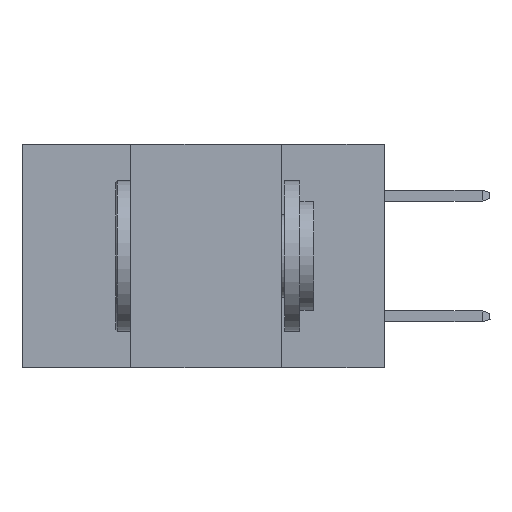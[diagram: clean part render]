
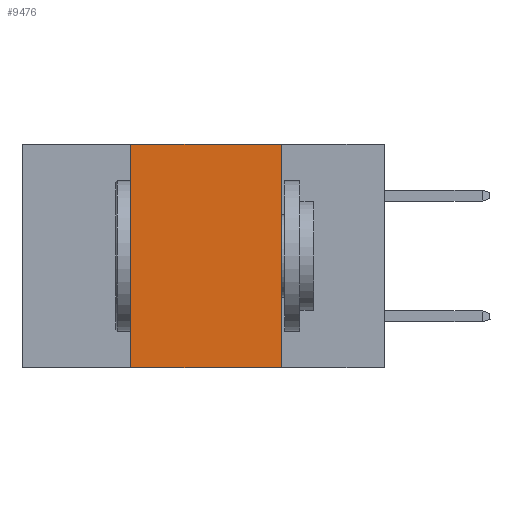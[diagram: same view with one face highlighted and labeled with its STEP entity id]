
A CAD part, left-side view. The second image highlights one B-rep face of the part: STEP entity #9476.
In plain terms, the highlighted planar face has unit normal (-1, 0, 0).
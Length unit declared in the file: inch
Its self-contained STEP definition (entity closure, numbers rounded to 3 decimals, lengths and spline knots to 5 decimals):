
#502 = LINE ( 'NONE', #11424, #1044 ) ;
#823 = LINE ( 'NONE', #8475, #12743 ) ;
#1044 = VECTOR ( 'NONE', #18278, 39.37008 ) ;
#2235 = EDGE_LOOP ( 'NONE', ( #3804, #17294, #13822, #14359 ) ) ;
#2372 = LINE ( 'NONE', #19545, #19688 ) ;
#2536 = CARTESIAN_POINT ( 'NONE',  ( 0., 0.6, -0.37 ) ) ;
#3804 = ORIENTED_EDGE ( 'NONE', *, *, #9839, .F. ) ;
#5320 = EDGE_CURVE ( 'NONE', #14919, #21281, #20371, .T. ) ;
#6186 = DIRECTION ( 'NONE',  ( 0., 0., -1. ) ) ;
#6721 = CARTESIAN_POINT ( 'NONE',  ( 0., 0.42, 0. ) ) ;
#7597 = EDGE_CURVE ( 'NONE', #14919, #21247, #823, .T. ) ;
#8021 = VERTEX_POINT ( 'NONE', #18153 ) ;
#8411 = DIRECTION ( 'NONE',  ( 0., 0., 1. ) ) ;
#8422 = CARTESIAN_POINT ( 'NONE',  ( 0., 0.17, -0.37 ) ) ;
#8475 = CARTESIAN_POINT ( 'NONE',  ( 0., 0.42, -0.37 ) ) ;
#8713 = PLANE ( 'NONE',  #11821 ) ;
#8721 = EDGE_CURVE ( 'NONE', #21247, #8021, #502, .T. ) ;
#9476 = ADVANCED_FACE ( 'NONE', ( #9817 ), #8713, .F. ) ;
#9817 = FACE_OUTER_BOUND ( 'NONE', #2235, .T. ) ;
#9839 = EDGE_CURVE ( 'NONE', #8021, #21281, #2372, .T. ) ;
#10393 = DIRECTION ( 'NONE',  ( 0., 0., -1. ) ) ;
#11424 = CARTESIAN_POINT ( 'NONE',  ( 0., 0.6, 0. ) ) ;
#11821 = AXIS2_PLACEMENT_3D ( 'NONE', #13675, #20328, #10393 ) ;
#12743 = VECTOR ( 'NONE', #8411, 39.37008 ) ;
#13665 = CARTESIAN_POINT ( 'NONE',  ( 0., 0.42, -0.37 ) ) ;
#13675 = CARTESIAN_POINT ( 'NONE',  ( 0., 0.6, 0. ) ) ;
#13822 = ORIENTED_EDGE ( 'NONE', *, *, #7597, .F. ) ;
#14359 = ORIENTED_EDGE ( 'NONE', *, *, #5320, .T. ) ;
#14919 = VERTEX_POINT ( 'NONE', #13665 ) ;
#16057 = VECTOR ( 'NONE', #19348, 39.37008 ) ;
#17294 = ORIENTED_EDGE ( 'NONE', *, *, #8721, .F. ) ;
#18153 = CARTESIAN_POINT ( 'NONE',  ( 0., 0.17, 0. ) ) ;
#18278 = DIRECTION ( 'NONE',  ( 0., -1., 0. ) ) ;
#19348 = DIRECTION ( 'NONE',  ( 0., -1., 0. ) ) ;
#19545 = CARTESIAN_POINT ( 'NONE',  ( 0., 0.17, -0.37 ) ) ;
#19688 = VECTOR ( 'NONE', #6186, 39.37008 ) ;
#20328 = DIRECTION ( 'NONE',  ( 1., 0., 0. ) ) ;
#20371 = LINE ( 'NONE', #2536, #16057 ) ;
#21247 = VERTEX_POINT ( 'NONE', #6721 ) ;
#21281 = VERTEX_POINT ( 'NONE', #8422 ) ;
